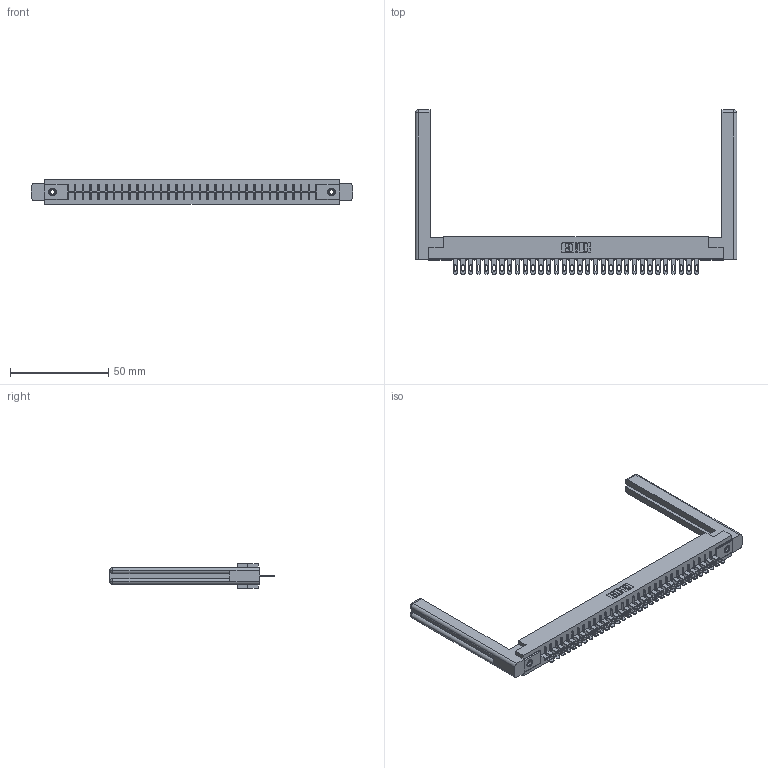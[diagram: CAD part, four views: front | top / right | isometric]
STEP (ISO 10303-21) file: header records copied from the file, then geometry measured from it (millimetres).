
FILE_DESCRIPTION (( 'STEP AP203' ), '1' );
FILE_NAME ('356-032-500-158.STEP', '2018-08-01T21:13:28', ( '' ), ( '' ), 'SwSTEP 2.0', 'SolidWorks 2016', '' );
FILE_SCHEMA (( 'CONFIG_CONTROL_DESIGN' ));
Length unit declared in the file: inch
Products named in the file (5): 307-220-058; 356-032-500-158; 306 Part_.156 Dia; 306-290-001_100; 345-250-001_345-250-001-102
Assembly tree (37 placements, depth 2):
  356-032-500-158
    306 Part_.156 Dia
    306-290-001_100  x32
    345-250-001_345-250-001-102  x2
    307-220-058  x2
Bounding box: 163.42 x 83.52 x 12.7 mm (x, y, z)
Volume: 25153.7 mm3; surface area: 24142.6 mm2
Topology: 37 solids, 37 shells, 2690 faces, 7550 edges, 4848 vertices
Faces by surface type: plane 1752, cylinder 786, sphere 128, cone 12, torus 12
Entity records: 33934 total; most frequent: CARTESIAN_POINT 5706, ORIENTED_EDGE 5598, DIRECTION 5583, EDGE_CURVE 2799, VECTOR 2177, LINE 2177, VERTEX_POINT 1772, AXIS2_PLACEMENT_3D 1703
